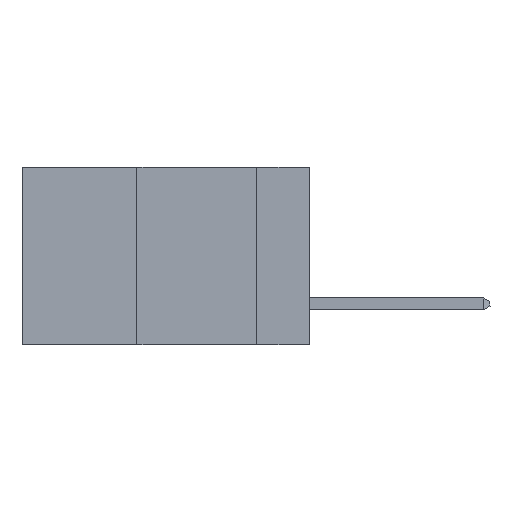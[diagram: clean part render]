
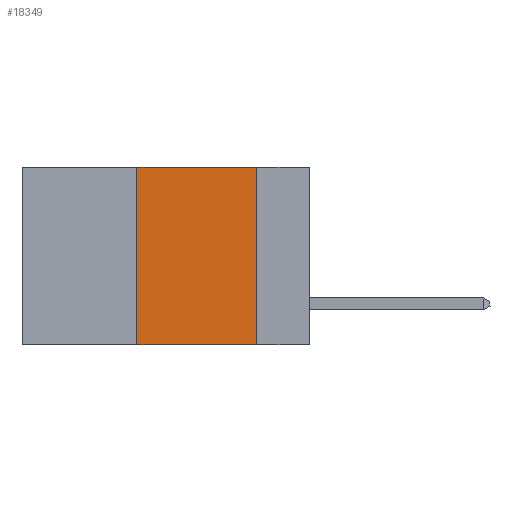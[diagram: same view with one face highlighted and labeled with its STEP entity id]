
A CAD part, left-side view. The second image highlights one B-rep face of the part: STEP entity #18349.
In plain terms, the highlighted planar face has unit normal (-1, 0, 0).
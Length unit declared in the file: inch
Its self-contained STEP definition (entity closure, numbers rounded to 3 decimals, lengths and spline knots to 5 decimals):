
#549 = EDGE_CURVE ( 'NONE', #9968, #12169, #6843, .T. ) ;
#609 = FACE_OUTER_BOUND ( 'NONE', #12678, .T. ) ;
#680 = ORIENTED_EDGE ( 'NONE', *, *, #16601, .F. ) ;
#735 = DIRECTION ( 'NONE',  ( 0., -1., 0. ) ) ;
#1700 = VECTOR ( 'NONE', #2823, 39.37008 ) ;
#1742 = ORIENTED_EDGE ( 'NONE', *, *, #7240, .T. ) ;
#1868 = CARTESIAN_POINT ( 'NONE',  ( 0., 0.36, -0.37 ) ) ;
#1975 = VERTEX_POINT ( 'NONE', #3737 ) ;
#2530 = LINE ( 'NONE', #8612, #18336 ) ;
#2822 = DIRECTION ( 'NONE',  ( 0., 0., -1. ) ) ;
#2823 = DIRECTION ( 'NONE',  ( 0., 0., 1. ) ) ;
#3737 = CARTESIAN_POINT ( 'NONE',  ( 0., 0.36, 0. ) ) ;
#3827 = CARTESIAN_POINT ( 'NONE',  ( 0., 0.11, -0.37 ) ) ;
#4105 = CARTESIAN_POINT ( 'NONE',  ( 0., 0.6, 0. ) ) ;
#5965 = VECTOR ( 'NONE', #14811, 39.37008 ) ;
#6843 = LINE ( 'NONE', #7434, #14483 ) ;
#7240 = EDGE_CURVE ( 'NONE', #13300, #12169, #2530, .T. ) ;
#7434 = CARTESIAN_POINT ( 'NONE',  ( 0., 0.11, 0. ) ) ;
#8597 = DIRECTION ( 'NONE',  ( 0., 0., -1. ) ) ;
#8612 = CARTESIAN_POINT ( 'NONE',  ( 0., 0.6, -0.37 ) ) ;
#9382 = EDGE_CURVE ( 'NONE', #13300, #1975, #18035, .T. ) ;
#9968 = VERTEX_POINT ( 'NONE', #10329 ) ;
#10329 = CARTESIAN_POINT ( 'NONE',  ( 0., 0.11, 0. ) ) ;
#10486 = CARTESIAN_POINT ( 'NONE',  ( 0., 0.6, 0. ) ) ;
#12031 = DIRECTION ( 'NONE',  ( 1., 0., 0. ) ) ;
#12169 = VERTEX_POINT ( 'NONE', #3827 ) ;
#12620 = ORIENTED_EDGE ( 'NONE', *, *, #549, .F. ) ;
#12678 = EDGE_LOOP ( 'NONE', ( #12620, #680, #17588, #1742 ) ) ;
#13300 = VERTEX_POINT ( 'NONE', #1868 ) ;
#14273 = AXIS2_PLACEMENT_3D ( 'NONE', #10486, #12031, #2822 ) ;
#14483 = VECTOR ( 'NONE', #8597, 39.37008 ) ;
#14811 = DIRECTION ( 'NONE',  ( 0., -1., 0. ) ) ;
#15093 = CARTESIAN_POINT ( 'NONE',  ( 0., 0.36, 0. ) ) ;
#16546 = PLANE ( 'NONE',  #14273 ) ;
#16601 = EDGE_CURVE ( 'NONE', #1975, #9968, #17606, .T. ) ;
#17588 = ORIENTED_EDGE ( 'NONE', *, *, #9382, .F. ) ;
#17606 = LINE ( 'NONE', #4105, #5965 ) ;
#18035 = LINE ( 'NONE', #15093, #1700 ) ;
#18336 = VECTOR ( 'NONE', #735, 39.37008 ) ;
#18349 = ADVANCED_FACE ( 'NONE', ( #609 ), #16546, .F. ) ;
